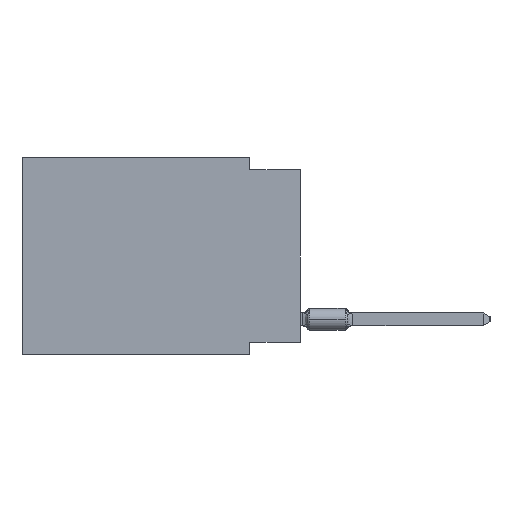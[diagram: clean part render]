
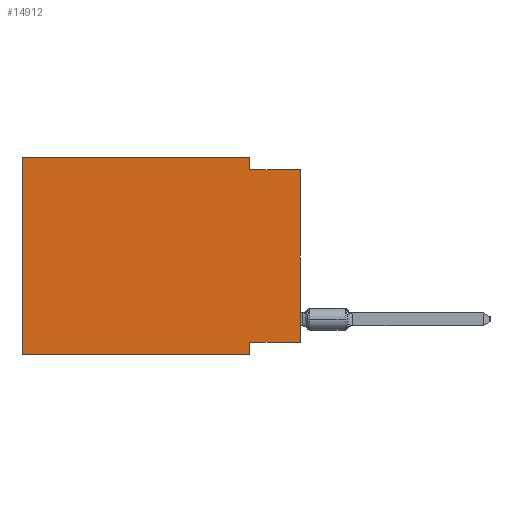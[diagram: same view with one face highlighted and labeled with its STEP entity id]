
A CAD part, left-side view. The second image highlights one B-rep face of the part: STEP entity #14912.
In plain terms, the highlighted planar face has unit normal (-1, 0, 0).
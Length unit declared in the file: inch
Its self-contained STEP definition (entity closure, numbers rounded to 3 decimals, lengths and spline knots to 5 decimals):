
#532 = VECTOR ( 'NONE', #37313, 39.37008 ) ;
#2206 = LINE ( 'NONE', #46375, #24059 ) ;
#2339 = VERTEX_POINT ( 'NONE', #16884 ) ;
#2652 = ORIENTED_EDGE ( 'NONE', *, *, #44251, .F. ) ;
#4817 = LINE ( 'NONE', #48270, #12300 ) ;
#4986 = VECTOR ( 'NONE', #11626, 39.37008 ) ;
#5455 = CARTESIAN_POINT ( 'NONE',  ( 0., 0.55, 0. ) ) ;
#5671 = DIRECTION ( 'NONE',  ( 0., 0., -1. ) ) ;
#5715 = AXIS2_PLACEMENT_3D ( 'NONE', #6535, #70663, #5671 ) ;
#6425 = CARTESIAN_POINT ( 'NONE',  ( 0., 0.1, -0.365 ) ) ;
#6535 = CARTESIAN_POINT ( 'NONE',  ( 0., 0.55, 0. ) ) ;
#11626 = DIRECTION ( 'NONE',  ( 0., -1., 0. ) ) ;
#12279 = CARTESIAN_POINT ( 'NONE',  ( 0., 0.55, -0.39 ) ) ;
#12300 = VECTOR ( 'NONE', #15981, 39.37008 ) ;
#14540 = VERTEX_POINT ( 'NONE', #62410 ) ;
#14912 = ADVANCED_FACE ( 'NONE', ( #71094 ), #51550, .F. ) ;
#15981 = DIRECTION ( 'NONE',  ( 0., -1., 0. ) ) ;
#16884 = CARTESIAN_POINT ( 'NONE',  ( 0., 0.1, -0.39 ) ) ;
#18095 = VERTEX_POINT ( 'NONE', #23156 ) ;
#18625 = LINE ( 'NONE', #5455, #532 ) ;
#18939 = CARTESIAN_POINT ( 'NONE',  ( 0., 0.1, -0.39 ) ) ;
#19079 = LINE ( 'NONE', #12279, #22286 ) ;
#19816 = EDGE_CURVE ( 'NONE', #14540, #18095, #4817, .T. ) ;
#21754 = CARTESIAN_POINT ( 'NONE',  ( 0., 0., -0.025 ) ) ;
#22286 = VECTOR ( 'NONE', #56501, 39.37008 ) ;
#23156 = CARTESIAN_POINT ( 'NONE',  ( 0., 0.1, 0. ) ) ;
#23682 = LINE ( 'NONE', #49599, #37624 ) ;
#24054 = DIRECTION ( 'NONE',  ( 0., 0., -1. ) ) ;
#24059 = VECTOR ( 'NONE', #73127, 39.37008 ) ;
#24340 = VERTEX_POINT ( 'NONE', #6425 ) ;
#25555 = VECTOR ( 'NONE', #47372, 39.37008 ) ;
#27118 = CARTESIAN_POINT ( 'NONE',  ( 0., 0., -0.365 ) ) ;
#29190 = EDGE_CURVE ( 'NONE', #41001, #51824, #23682, .T. ) ;
#36648 = ORIENTED_EDGE ( 'NONE', *, *, #40894, .T. ) ;
#37313 = DIRECTION ( 'NONE',  ( 0., 0., 1. ) ) ;
#37624 = VECTOR ( 'NONE', #67881, 39.37008 ) ;
#40894 = EDGE_CURVE ( 'NONE', #52562, #2339, #19079, .T. ) ;
#41001 = VERTEX_POINT ( 'NONE', #27118 ) ;
#42463 = EDGE_CURVE ( 'NONE', #18095, #44178, #2206, .T. ) ;
#44178 = VERTEX_POINT ( 'NONE', #49771 ) ;
#44251 = EDGE_CURVE ( 'NONE', #41001, #24340, #66087, .T. ) ;
#46375 = CARTESIAN_POINT ( 'NONE',  ( 0., 0.1, 0. ) ) ;
#47372 = DIRECTION ( 'NONE',  ( 0., 1., 0. ) ) ;
#48270 = CARTESIAN_POINT ( 'NONE',  ( 0., 0.55, 0. ) ) ;
#49599 = CARTESIAN_POINT ( 'NONE',  ( 0., 0., 0. ) ) ;
#49771 = CARTESIAN_POINT ( 'NONE',  ( 0., 0.1, -0.025 ) ) ;
#51550 = PLANE ( 'NONE',  #5715 ) ;
#51824 = VERTEX_POINT ( 'NONE', #21754 ) ;
#52101 = EDGE_CURVE ( 'NONE', #52562, #14540, #18625, .T. ) ;
#52562 = VERTEX_POINT ( 'NONE', #75496 ) ;
#54248 = ORIENTED_EDGE ( 'NONE', *, *, #42463, .F. ) ;
#55916 = ORIENTED_EDGE ( 'NONE', *, *, #82052, .F. ) ;
#56501 = DIRECTION ( 'NONE',  ( 0., -1., 0. ) ) ;
#58259 = ORIENTED_EDGE ( 'NONE', *, *, #52101, .F. ) ;
#59697 = ORIENTED_EDGE ( 'NONE', *, *, #19816, .F. ) ;
#60062 = ORIENTED_EDGE ( 'NONE', *, *, #29190, .T. ) ;
#60548 = CARTESIAN_POINT ( 'NONE',  ( 0., 0., -0.365 ) ) ;
#60903 = EDGE_CURVE ( 'NONE', #24340, #2339, #69505, .T. ) ;
#62410 = CARTESIAN_POINT ( 'NONE',  ( 0., 0.55, 0. ) ) ;
#63041 = CARTESIAN_POINT ( 'NONE',  ( 0., 0., -0.025 ) ) ;
#65209 = VECTOR ( 'NONE', #24054, 39.37008 ) ;
#66087 = LINE ( 'NONE', #60548, #25555 ) ;
#67881 = DIRECTION ( 'NONE',  ( 0., 0., 1. ) ) ;
#69505 = LINE ( 'NONE', #18939, #65209 ) ;
#70536 = EDGE_LOOP ( 'NONE', ( #60062, #55916, #54248, #59697, #58259, #36648, #76191, #2652 ) ) ;
#70663 = DIRECTION ( 'NONE',  ( 1., 0., 0. ) ) ;
#71094 = FACE_OUTER_BOUND ( 'NONE', #70536, .T. ) ;
#73127 = DIRECTION ( 'NONE',  ( 0., 0., -1. ) ) ;
#75496 = CARTESIAN_POINT ( 'NONE',  ( 0., 0.55, -0.39 ) ) ;
#76191 = ORIENTED_EDGE ( 'NONE', *, *, #60903, .F. ) ;
#82052 = EDGE_CURVE ( 'NONE', #44178, #51824, #83429, .T. ) ;
#83429 = LINE ( 'NONE', #63041, #4986 ) ;
